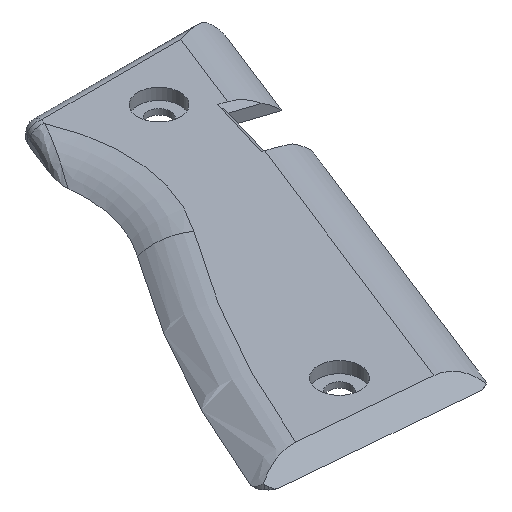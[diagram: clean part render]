
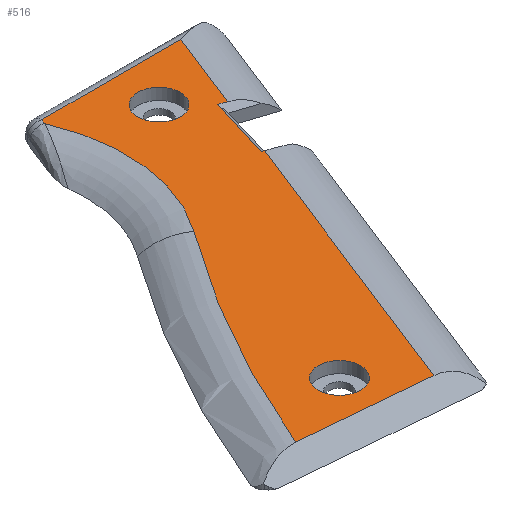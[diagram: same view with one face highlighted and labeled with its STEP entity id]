
A CAD part, isometric view. The second image highlights one B-rep face of the part: STEP entity #516.
In plain terms, the highlighted planar face has unit normal (0, 0, 1).
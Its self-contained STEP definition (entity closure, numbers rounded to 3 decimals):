
#19=FACE_BOUND('',#178,.T.);
#20=FACE_BOUND('',#179,.T.);
#28=PLANE('',#579);
#39=LINE('',#823,#75);
#41=LINE('',#838,#77);
#54=LINE('',#886,#90);
#58=LINE('',#934,#94);
#59=LINE('',#936,#95);
#60=LINE('',#938,#96);
#61=LINE('',#940,#97);
#62=LINE('',#941,#98);
#75=VECTOR('',#620,10.);
#77=VECTOR('',#630,10.);
#90=VECTOR('',#673,10.);
#94=VECTOR('',#695,10.);
#95=VECTOR('',#696,10.);
#96=VECTOR('',#697,10.);
#97=VECTOR('',#698,10.);
#98=VECTOR('',#699,10.);
#144=FACE_OUTER_BOUND('',#177,.T.);
#177=EDGE_LOOP('',(#421,#422,#423,#424,#425,#426,#427,#428,#429,#430));
#178=EDGE_LOOP('',(#431));
#179=EDGE_LOOP('',(#432));
#213=CIRCLE('',#578,198.609);
#214=CIRCLE('',#580,30.133);
#215=CIRCLE('',#581,3.75);
#216=CIRCLE('',#582,3.75);
#232=VERTEX_POINT('',#801);
#237=VERTEX_POINT('',#820);
#238=VERTEX_POINT('',#822);
#258=VERTEX_POINT('',#883);
#259=VERTEX_POINT('',#885);
#263=VERTEX_POINT('',#919);
#264=VERTEX_POINT('',#933);
#265=VERTEX_POINT('',#935);
#266=VERTEX_POINT('',#937);
#267=VERTEX_POINT('',#939);
#268=VERTEX_POINT('',#942);
#269=VERTEX_POINT('',#944);
#285=EDGE_CURVE('',#237,#238,#39,.T.);
#290=EDGE_CURVE('',#232,#237,#41,.T.);
#313=EDGE_CURVE('',#258,#259,#54,.T.);
#322=EDGE_CURVE('',#259,#263,#213,.T.);
#324=EDGE_CURVE('',#263,#232,#214,.T.);
#325=EDGE_CURVE('',#264,#258,#58,.T.);
#326=EDGE_CURVE('',#265,#264,#59,.T.);
#327=EDGE_CURVE('',#266,#265,#60,.T.);
#328=EDGE_CURVE('',#267,#266,#61,.T.);
#329=EDGE_CURVE('',#238,#267,#62,.T.);
#330=EDGE_CURVE('',#268,#268,#215,.F.);
#331=EDGE_CURVE('',#269,#269,#216,.F.);
#421=ORIENTED_EDGE('',*,*,#290,.F.);
#422=ORIENTED_EDGE('',*,*,#324,.F.);
#423=ORIENTED_EDGE('',*,*,#322,.F.);
#424=ORIENTED_EDGE('',*,*,#313,.F.);
#425=ORIENTED_EDGE('',*,*,#325,.F.);
#426=ORIENTED_EDGE('',*,*,#326,.F.);
#427=ORIENTED_EDGE('',*,*,#327,.F.);
#428=ORIENTED_EDGE('',*,*,#328,.F.);
#429=ORIENTED_EDGE('',*,*,#329,.F.);
#430=ORIENTED_EDGE('',*,*,#285,.F.);
#431=ORIENTED_EDGE('',*,*,#330,.T.);
#432=ORIENTED_EDGE('',*,*,#331,.T.);
#516=ADVANCED_FACE('',(#144,#19,#20),#28,.F.);
#578=AXIS2_PLACEMENT_3D('',#920,#689,#690);
#579=AXIS2_PLACEMENT_3D('',#931,#691,#692);
#580=AXIS2_PLACEMENT_3D('',#932,#693,#694);
#581=AXIS2_PLACEMENT_3D('',#943,#700,#701);
#582=AXIS2_PLACEMENT_3D('',#945,#702,#703);
#620=DIRECTION('',(1.,0.,0.));
#630=DIRECTION('',(0.367,0.93,0.));
#673=DIRECTION('',(-0.996,0.089,0.));
#689=DIRECTION('center_axis',(0.,0.,-1.));
#690=DIRECTION('ref_axis',(0.874,-0.486,0.));
#691=DIRECTION('center_axis',(0.,0.,-1.));
#692=DIRECTION('ref_axis',(1.,0.,0.));
#693=DIRECTION('center_axis',(0.,0.,1.));
#694=DIRECTION('ref_axis',(-0.974,0.228,0.));
#695=DIRECTION('',(-0.367,-0.93,0.));
#696=DIRECTION('',(0.951,-0.31,0.));
#697=DIRECTION('',(-0.292,-0.956,0.));
#698=DIRECTION('',(-0.951,0.31,0.));
#699=DIRECTION('',(-0.367,-0.93,0.));
#700=DIRECTION('center_axis',(0.,0.,1.));
#701=DIRECTION('ref_axis',(-1.,0.,0.));
#702=DIRECTION('center_axis',(0.,0.,1.));
#703=DIRECTION('ref_axis',(-1.,0.,0.));
#801=CARTESIAN_POINT('',(76.169,-15.911,16.9));
#820=CARTESIAN_POINT('',(76.503,-15.063,16.9));
#822=CARTESIAN_POINT('',(101.013,-15.063,16.9));
#823=CARTESIAN_POINT('',(80.438,-15.063,16.9));
#838=CARTESIAN_POINT('',(69.703,-32.326,16.9));
#883=CARTESIAN_POINT('',(71.983,-88.759,16.9));
#885=CARTESIAN_POINT('',(49.624,-86.762,16.9));
#886=CARTESIAN_POINT('',(78.853,-89.372,16.9));
#919=CARTESIAN_POINT('',(72.861,-45.542,16.9));
#920=CARTESIAN_POINT('Origin',(233.022,-162.989,16.9));
#931=CARTESIAN_POINT('Origin',(84.373,-48.148,16.9));
#932=CARTESIAN_POINT('Origin',(48.489,-27.821,16.9));
#933=CARTESIAN_POINT('',(91.408,-39.446,16.9));
#934=CARTESIAN_POINT('',(94.693,-31.108,16.9));
#935=CARTESIAN_POINT('',(90.956,-39.299,16.9));
#936=CARTESIAN_POINT('',(89.752,-38.906,16.9));
#937=CARTESIAN_POINT('',(94.317,-28.281,16.9));
#938=CARTESIAN_POINT('',(90.972,-39.244,16.9));
#939=CARTESIAN_POINT('',(95.637,-28.712,16.9));
#940=CARTESIAN_POINT('',(96.784,-29.086,16.9));
#941=CARTESIAN_POINT('',(94.693,-31.108,16.9));
#942=CARTESIAN_POINT('',(92.882,-23.118,16.9));
#943=CARTESIAN_POINT('Origin',(89.132,-23.118,16.9));
#944=CARTESIAN_POINT('',(67.042,-80.791,16.9));
#945=CARTESIAN_POINT('Origin',(63.292,-80.791,16.9));
